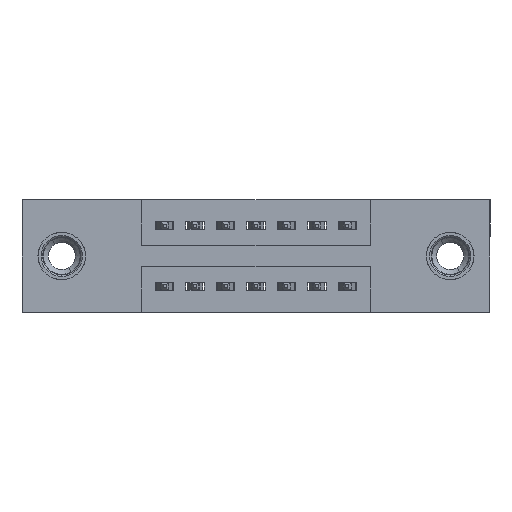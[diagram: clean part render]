
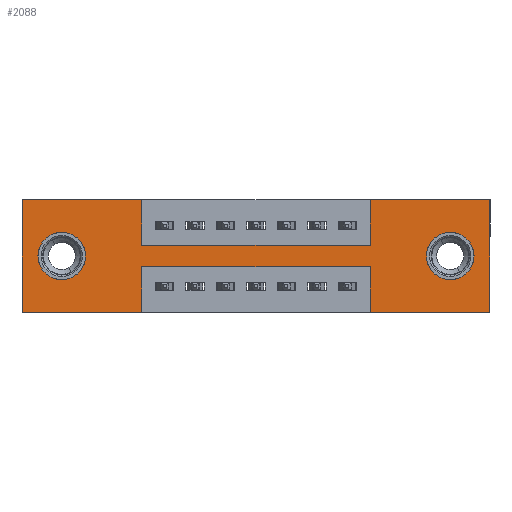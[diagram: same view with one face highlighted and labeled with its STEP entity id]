
A CAD part, front view. The second image highlights one B-rep face of the part: STEP entity #2088.
In plain terms, the highlighted planar face has unit normal (0, -1, 0).
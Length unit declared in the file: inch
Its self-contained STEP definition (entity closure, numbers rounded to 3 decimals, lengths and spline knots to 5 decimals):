
#69 = VERTEX_POINT ( 'NONE', #10094 ) ;
#192 = CARTESIAN_POINT ( 'NONE',  ( 0.3925, 0., -0.37 ) ) ;
#259 = DIRECTION ( 'NONE',  ( -1., 0., 0. ) ) ;
#384 = CARTESIAN_POINT ( 'NONE',  ( 0.3925, 0., -0.37 ) ) ;
#397 = DIRECTION ( 'NONE',  ( 0., 0., -1. ) ) ;
#452 = VERTEX_POINT ( 'NONE', #6769 ) ;
#661 = VECTOR ( 'NONE', #9502, 39.37008 ) ;
#663 = CARTESIAN_POINT ( 'NONE',  ( 1.1425, 0., -0.37 ) ) ;
#926 = DIRECTION ( 'NONE',  ( 0., 0., 1. ) ) ;
#973 = EDGE_CURVE ( 'NONE', #14507, #5758, #6140, .T. ) ;
#999 = AXIS2_PLACEMENT_3D ( 'NONE', #10801, #12365, #926 ) ;
#1083 = VERTEX_POINT ( 'NONE', #384 ) ;
#1175 = EDGE_CURVE ( 'NONE', #12732, #7934, #5942, .T. ) ;
#1305 = CARTESIAN_POINT ( 'NONE',  ( 0.3925, 0., -0.15 ) ) ;
#1428 = CIRCLE ( 'NONE', #999, 0.078 ) ;
#1570 = ORIENTED_EDGE ( 'NONE', *, *, #7278, .F. ) ;
#1652 = EDGE_LOOP ( 'NONE', ( #14028, #13287 ) ) ;
#1678 = VERTEX_POINT ( 'NONE', #6586 ) ;
#2080 = EDGE_CURVE ( 'NONE', #5758, #8515, #12272, .T. ) ;
#2088 = ADVANCED_FACE ( 'NONE', ( #11515, #11146, #5405 ), #2834, .T. ) ;
#2354 = VECTOR ( 'NONE', #12013, 39.37008 ) ;
#2429 = VECTOR ( 'NONE', #259, 39.37008 ) ;
#2447 = AXIS2_PLACEMENT_3D ( 'NONE', #11669, #12865, #4931 ) ;
#2678 = DIRECTION ( 'NONE',  ( 0., 0., -1. ) ) ;
#2699 = LINE ( 'NONE', #2700, #2354 ) ;
#2700 = CARTESIAN_POINT ( 'NONE',  ( 0.3925, 0., 0. ) ) ;
#2758 = CARTESIAN_POINT ( 'NONE',  ( 1.405, 0., -0.107 ) ) ;
#2834 = PLANE ( 'NONE',  #12424 ) ;
#2853 = ORIENTED_EDGE ( 'NONE', *, *, #14398, .F. ) ;
#3056 = CARTESIAN_POINT ( 'NONE',  ( 0., 0., 0. ) ) ;
#3097 = VECTOR ( 'NONE', #5928, 39.37008 ) ;
#3314 = VERTEX_POINT ( 'NONE', #12437 ) ;
#3324 = DIRECTION ( 'NONE',  ( 0., 1., 0. ) ) ;
#3385 = AXIS2_PLACEMENT_3D ( 'NONE', #9693, #7276, #2678 ) ;
#3518 = ORIENTED_EDGE ( 'NONE', *, *, #3608, .F. ) ;
#3608 = EDGE_CURVE ( 'NONE', #6332, #11332, #3636, .T. ) ;
#3612 = VECTOR ( 'NONE', #12699, 39.37008 ) ;
#3636 = LINE ( 'NONE', #1305, #7535 ) ;
#3797 = LINE ( 'NONE', #10406, #3612 ) ;
#3867 = DIRECTION ( 'NONE',  ( 0., 0., -1. ) ) ;
#3888 = LINE ( 'NONE', #7131, #2429 ) ;
#4153 = ORIENTED_EDGE ( 'NONE', *, *, #4311, .F. ) ;
#4246 = DIRECTION ( 'NONE',  ( 0., 0., 1. ) ) ;
#4311 = EDGE_CURVE ( 'NONE', #7934, #69, #3797, .T. ) ;
#4355 = AXIS2_PLACEMENT_3D ( 'NONE', #6801, #3324, #13925 ) ;
#4455 = ORIENTED_EDGE ( 'NONE', *, *, #10272, .F. ) ;
#4730 = CARTESIAN_POINT ( 'NONE',  ( 1.535, 0., 0. ) ) ;
#4931 = DIRECTION ( 'NONE',  ( 0., 0., 1. ) ) ;
#5297 = ORIENTED_EDGE ( 'NONE', *, *, #8404, .T. ) ;
#5367 = CARTESIAN_POINT ( 'NONE',  ( 1.405, 0., -0.263 ) ) ;
#5387 = LINE ( 'NONE', #192, #13543 ) ;
#5405 = FACE_OUTER_BOUND ( 'NONE', #13184, .T. ) ;
#5684 = EDGE_LOOP ( 'NONE', ( #5297, #7602 ) ) ;
#5758 = VERTEX_POINT ( 'NONE', #9071 ) ;
#5928 = DIRECTION ( 'NONE',  ( 1., 0., 0. ) ) ;
#5942 = LINE ( 'NONE', #9981, #6310 ) ;
#6140 = LINE ( 'NONE', #3056, #3097 ) ;
#6207 = CARTESIAN_POINT ( 'NONE',  ( 0., 0., -0.37 ) ) ;
#6289 = VERTEX_POINT ( 'NONE', #2758 ) ;
#6310 = VECTOR ( 'NONE', #4246, 39.37008 ) ;
#6332 = VERTEX_POINT ( 'NONE', #13181 ) ;
#6474 = EDGE_CURVE ( 'NONE', #3314, #1678, #11623, .T. ) ;
#6586 = CARTESIAN_POINT ( 'NONE',  ( 0.3925, 0., -0.22 ) ) ;
#6769 = CARTESIAN_POINT ( 'NONE',  ( 0.13, 0., -0.107 ) ) ;
#6801 = CARTESIAN_POINT ( 'NONE',  ( 1.405, 0., -0.185 ) ) ;
#6904 = VERTEX_POINT ( 'NONE', #5367 ) ;
#6991 = DIRECTION ( 'NONE',  ( 0., 0., -1. ) ) ;
#7131 = CARTESIAN_POINT ( 'NONE',  ( 0., 0., -0.37 ) ) ;
#7159 = DIRECTION ( 'NONE',  ( 0., 0., 1. ) ) ;
#7237 = CARTESIAN_POINT ( 'NONE',  ( 0.3925, 0., -0.22 ) ) ;
#7276 = DIRECTION ( 'NONE',  ( 0., 1., 0. ) ) ;
#7278 = EDGE_CURVE ( 'NONE', #1083, #12732, #3888, .T. ) ;
#7338 = EDGE_CURVE ( 'NONE', #6904, #6289, #10304, .T. ) ;
#7453 = ORIENTED_EDGE ( 'NONE', *, *, #10424, .F. ) ;
#7535 = VECTOR ( 'NONE', #11748, 39.37008 ) ;
#7589 = LINE ( 'NONE', #663, #9585 ) ;
#7602 = ORIENTED_EDGE ( 'NONE', *, *, #7338, .T. ) ;
#7934 = VERTEX_POINT ( 'NONE', #13597 ) ;
#8045 = CARTESIAN_POINT ( 'NONE',  ( 1.535, 0., -0.37 ) ) ;
#8074 = VERTEX_POINT ( 'NONE', #13115 ) ;
#8151 = VECTOR ( 'NONE', #9870, 39.37008 ) ;
#8373 = EDGE_CURVE ( 'NONE', #8074, #3314, #7589, .T. ) ;
#8404 = EDGE_CURVE ( 'NONE', #6289, #6904, #11771, .T. ) ;
#8515 = VERTEX_POINT ( 'NONE', #8045 ) ;
#8625 = LINE ( 'NONE', #11757, #13031 ) ;
#8910 = CARTESIAN_POINT ( 'NONE',  ( 0.13, 0., -0.263 ) ) ;
#8939 = CARTESIAN_POINT ( 'NONE',  ( 0., 0., -0.37 ) ) ;
#9071 = CARTESIAN_POINT ( 'NONE',  ( 1.535, 0., 0. ) ) ;
#9132 = VECTOR ( 'NONE', #6991, 39.37008 ) ;
#9490 = CARTESIAN_POINT ( 'NONE',  ( 0., 0., -0.37 ) ) ;
#9491 = ORIENTED_EDGE ( 'NONE', *, *, #1175, .F. ) ;
#9502 = DIRECTION ( 'NONE',  ( -1., 0., 0. ) ) ;
#9527 = VERTEX_POINT ( 'NONE', #8910 ) ;
#9585 = VECTOR ( 'NONE', #11915, 39.37008 ) ;
#9693 = CARTESIAN_POINT ( 'NONE',  ( 1.405, 0., -0.185 ) ) ;
#9870 = DIRECTION ( 'NONE',  ( -1., 0., 0. ) ) ;
#9981 = CARTESIAN_POINT ( 'NONE',  ( 0., 0., 0. ) ) ;
#10094 = CARTESIAN_POINT ( 'NONE',  ( 0.3925, 0., 0. ) ) ;
#10272 = EDGE_CURVE ( 'NONE', #11332, #14507, #8625, .T. ) ;
#10304 = CIRCLE ( 'NONE', #3385, 0.078 ) ;
#10406 = CARTESIAN_POINT ( 'NONE',  ( 0., 0., 0. ) ) ;
#10424 = EDGE_CURVE ( 'NONE', #69, #6332, #2699, .T. ) ;
#10704 = DIRECTION ( 'NONE',  ( 0., -1., 0. ) ) ;
#10735 = CIRCLE ( 'NONE', #2447, 0.078 ) ;
#10801 = CARTESIAN_POINT ( 'NONE',  ( 0.13, 0., -0.185 ) ) ;
#11146 = FACE_BOUND ( 'NONE', #1652, .T. ) ;
#11167 = EDGE_CURVE ( 'NONE', #9527, #452, #1428, .T. ) ;
#11332 = VERTEX_POINT ( 'NONE', #13632 ) ;
#11385 = CARTESIAN_POINT ( 'NONE',  ( 1.1425, 0., 0. ) ) ;
#11405 = ORIENTED_EDGE ( 'NONE', *, *, #973, .F. ) ;
#11515 = FACE_BOUND ( 'NONE', #5684, .T. ) ;
#11623 = LINE ( 'NONE', #7237, #661 ) ;
#11642 = EDGE_CURVE ( 'NONE', #1678, #1083, #5387, .T. ) ;
#11669 = CARTESIAN_POINT ( 'NONE',  ( 0.13, 0., -0.185 ) ) ;
#11731 = EDGE_CURVE ( 'NONE', #452, #9527, #10735, .T. ) ;
#11748 = DIRECTION ( 'NONE',  ( 1., 0., 0. ) ) ;
#11757 = CARTESIAN_POINT ( 'NONE',  ( 1.1425, 0., 0. ) ) ;
#11771 = CIRCLE ( 'NONE', #4355, 0.078 ) ;
#11915 = DIRECTION ( 'NONE',  ( 0., 0., 1. ) ) ;
#12013 = DIRECTION ( 'NONE',  ( 0., 0., -1. ) ) ;
#12272 = LINE ( 'NONE', #4730, #9132 ) ;
#12365 = DIRECTION ( 'NONE',  ( 0., 1., 0. ) ) ;
#12424 = AXIS2_PLACEMENT_3D ( 'NONE', #9490, #10704, #3867 ) ;
#12437 = CARTESIAN_POINT ( 'NONE',  ( 1.1425, 0., -0.22 ) ) ;
#12699 = DIRECTION ( 'NONE',  ( 1., 0., 0. ) ) ;
#12732 = VERTEX_POINT ( 'NONE', #8939 ) ;
#12865 = DIRECTION ( 'NONE',  ( 0., 1., 0. ) ) ;
#13031 = VECTOR ( 'NONE', #7159, 39.37008 ) ;
#13091 = LINE ( 'NONE', #6207, #8151 ) ;
#13115 = CARTESIAN_POINT ( 'NONE',  ( 1.1425, 0., -0.37 ) ) ;
#13181 = CARTESIAN_POINT ( 'NONE',  ( 0.3925, 0., -0.15 ) ) ;
#13184 = EDGE_LOOP ( 'NONE', ( #13341, #14622, #14312, #2853, #13490, #11405, #4455, #3518, #7453, #4153, #9491, #1570 ) ) ;
#13287 = ORIENTED_EDGE ( 'NONE', *, *, #11167, .T. ) ;
#13341 = ORIENTED_EDGE ( 'NONE', *, *, #11642, .F. ) ;
#13490 = ORIENTED_EDGE ( 'NONE', *, *, #2080, .F. ) ;
#13543 = VECTOR ( 'NONE', #397, 39.37008 ) ;
#13597 = CARTESIAN_POINT ( 'NONE',  ( 0., 0., 0. ) ) ;
#13632 = CARTESIAN_POINT ( 'NONE',  ( 1.1425, 0., -0.15 ) ) ;
#13925 = DIRECTION ( 'NONE',  ( 0., 0., -1. ) ) ;
#14028 = ORIENTED_EDGE ( 'NONE', *, *, #11731, .T. ) ;
#14312 = ORIENTED_EDGE ( 'NONE', *, *, #8373, .F. ) ;
#14398 = EDGE_CURVE ( 'NONE', #8515, #8074, #13091, .T. ) ;
#14507 = VERTEX_POINT ( 'NONE', #11385 ) ;
#14622 = ORIENTED_EDGE ( 'NONE', *, *, #6474, .F. ) ;
